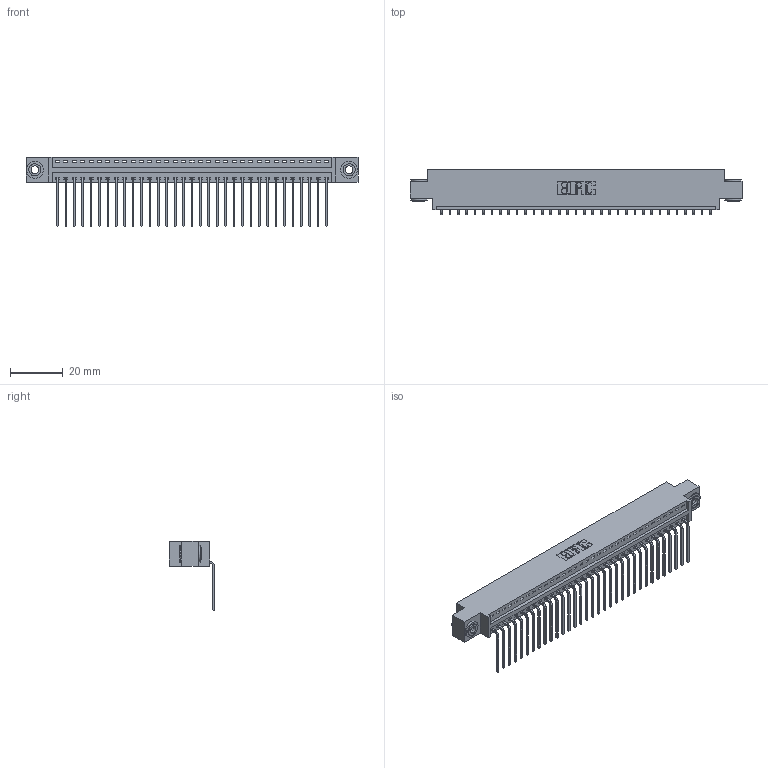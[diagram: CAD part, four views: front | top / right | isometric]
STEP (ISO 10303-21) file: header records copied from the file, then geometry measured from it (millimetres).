
FILE_DESCRIPTION (( 'STEP AP203' ), '1' );
FILE_NAME ('346-033-559-603.STEP', '2018-08-23T21:24:34', ( '' ), ( '' ), 'SwSTEP 2.0', 'SolidWorks 2016', '' );
FILE_SCHEMA (( 'CONFIG_CONTROL_DESIGN' ));
Length unit declared in the file: inch
Products named in the file (4): 345-250-002_345-250-002-102; 346-033-559-603; 346 Part_0.170 Offset - 0.156 Dia-TH; 345-292-001_558 559 Tail - 1
Assembly tree (36 placements, depth 2):
  346-033-559-603
    346 Part_0.170 Offset - 0.156 Dia-TH
    345-292-001_558 559 Tail - 1  x33
    345-250-002_345-250-002-102  x2
Bounding box: 125.35 x 17.08 x 26.16 mm (x, y, z)
Volume: 11911.4 mm3; surface area: 15826 mm2
Topology: 36 solids, 36 shells, 2144 faces, 6423 edges, 4234 vertices
Faces by surface type: plane 1476, cylinder 660, cone 8
Entity records: 22558 total; most frequent: CARTESIAN_POINT 3850, ORIENTED_EDGE 3810, DIRECTION 3437, EDGE_CURVE 1905, VECTOR 1617, LINE 1617, VERTEX_POINT 1266, AXIS2_PLACEMENT_3D 910
